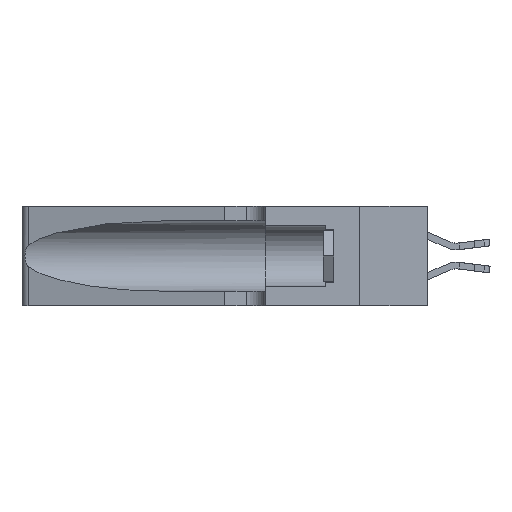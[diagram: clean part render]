
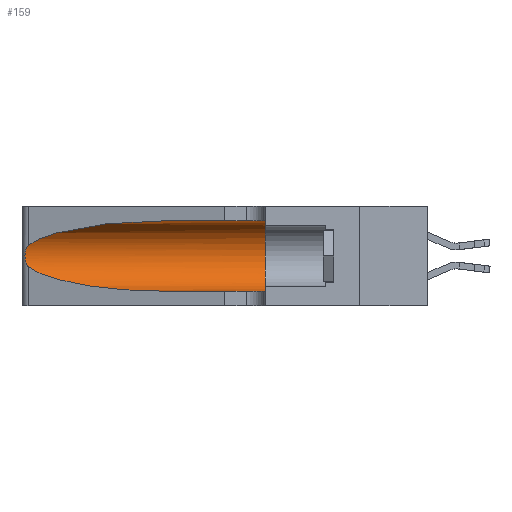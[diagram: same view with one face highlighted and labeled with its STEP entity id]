
A CAD part, left-side view. The second image highlights one B-rep face of the part: STEP entity #159.
In plain terms, the highlighted cylindrical face has radius 3.308 mm (diameter 6.617 mm), a partial arc.
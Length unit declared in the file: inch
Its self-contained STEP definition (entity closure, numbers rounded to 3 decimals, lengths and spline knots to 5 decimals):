
#159 = ADVANCED_FACE ( 'NONE', ( #13411 ), #8595, .F. ) ;
#199 = CARTESIAN_POINT ( 'NONE',  ( 0.1305, 0.35, 0.05475 ) ) ;
#634 = CARTESIAN_POINT ( 'NONE',  ( 0.26017, 1.23833, 0.17102 ) ) ;
#737 = CARTESIAN_POINT ( 'NONE',  ( 0.25487, 1.22718, 0.22369 ) ) ;
#1024 =( BOUNDED_CURVE ( )  B_SPLINE_CURVE ( 3, ( #13643, #17890, #12179, #4839 ),
 .UNSPECIFIED., .F., .T. ) 
 B_SPLINE_CURVE_WITH_KNOTS ( ( 4, 4 ),
 ( 3.44316, 4.71239 ),
 .UNSPECIFIED. ) 
 CURVE ( )  GEOMETRIC_REPRESENTATION_ITEM ( )  RATIONAL_B_SPLINE_CURVE ( ( 1., 0.87, 0.87, 1. ) ) 
 REPRESENTATION_ITEM ( '' )  );
#2103 = CARTESIAN_POINT ( 'NONE',  ( 0.25487, 1.22718, 0.22369 ) ) ;
#2173 = CARTESIAN_POINT ( 'NONE',  ( 0.25555, 1.22994, 0.2215 ) ) ;
#2237 = CARTESIAN_POINT ( 'NONE',  ( 0.25789, 1.23486, 0.15765 ) ) ;
#2696 = EDGE_CURVE ( 'NONE', #3798, #12055, #2937, .T. ) ;
#2868 = DIRECTION ( 'NONE',  ( 0., 1., 0. ) ) ;
#2937 =( BOUNDED_CURVE ( )  B_SPLINE_CURVE ( 3, ( #15737, #5533, #4028, #7050 ),
 .UNSPECIFIED., .F., .F. ) 
 B_SPLINE_CURVE_WITH_KNOTS ( ( 4, 4 ),
 ( 1.5708, 2.84003 ),
 .UNSPECIFIED. ) 
 CURVE ( )  GEOMETRIC_REPRESENTATION_ITEM ( )  RATIONAL_B_SPLINE_CURVE ( ( 1., 0.87, 0.87, 1. ) ) 
 REPRESENTATION_ITEM ( '' )  );
#3325 = VECTOR ( 'NONE', #5271, 39.37008 ) ;
#3624 = EDGE_CURVE ( 'NONE', #12443, #8370, #1024, .T. ) ;
#3798 = VERTEX_POINT ( 'NONE', #6885 ) ;
#3834 = CARTESIAN_POINT ( 'NONE',  ( 0.25555, 1.22993, 0.14849 ) ) ;
#4028 = CARTESIAN_POINT ( 'NONE',  ( 0.2373, 1.15595, 0.28018 ) ) ;
#4427 = EDGE_CURVE ( 'NONE', #12055, #12443, #14696, .T. ) ;
#4839 = CARTESIAN_POINT ( 'NONE',  ( 0.1305, 0.72297, 0.05475 ) ) ;
#5271 = DIRECTION ( 'NONE',  ( 0., -1., 0. ) ) ;
#5533 = CARTESIAN_POINT ( 'NONE',  ( 0.18966, 0.96281, 0.31525 ) ) ;
#5988 = AXIS2_PLACEMENT_3D ( 'NONE', #7553, #13206, #16961 ) ;
#6084 = CARTESIAN_POINT ( 'NONE',  ( 0.1305, 1.61858, 0.05475 ) ) ;
#6460 = EDGE_CURVE ( 'NONE', #8370, #10790, #11278, .T. ) ;
#6661 = ORIENTED_EDGE ( 'NONE', *, *, #2696, .T. ) ;
#6793 = CARTESIAN_POINT ( 'NONE',  ( 0.25787, 1.23484, 0.2124 ) ) ;
#6885 = CARTESIAN_POINT ( 'NONE',  ( 0.1305, 0.72297, 0.31525 ) ) ;
#6924 = ORIENTED_EDGE ( 'NONE', *, *, #4427, .T. ) ;
#6976 = ORIENTED_EDGE ( 'NONE', *, *, #3624, .T. ) ;
#7050 = CARTESIAN_POINT ( 'NONE',  ( 0.25487, 1.22718, 0.22369 ) ) ;
#7472 = AXIS2_PLACEMENT_3D ( 'NONE', #11776, #2868, #13247 ) ;
#7485 = ORIENTED_EDGE ( 'NONE', *, *, #8399, .F. ) ;
#7553 = CARTESIAN_POINT ( 'NONE',  ( 0.1305, 1.61858, 0.185 ) ) ;
#7874 = ORIENTED_EDGE ( 'NONE', *, *, #6460, .T. ) ;
#7990 = ORIENTED_EDGE ( 'NONE', *, *, #12810, .F. ) ;
#8241 = CARTESIAN_POINT ( 'NONE',  ( 0.26018, 1.23835, 0.19895 ) ) ;
#8370 = VERTEX_POINT ( 'NONE', #18313 ) ;
#8399 = EDGE_CURVE ( 'NONE', #3798, #17094, #15078, .T. ) ;
#8595 = CYLINDRICAL_SURFACE ( 'NONE', #5988, 0.13025 ) ;
#9730 = CARTESIAN_POINT ( 'NONE',  ( 0.26075, 1.23896, 0.178 ) ) ;
#10790 = VERTEX_POINT ( 'NONE', #199 ) ;
#10812 = VECTOR ( 'NONE', #17688, 39.37008 ) ;
#11194 = CARTESIAN_POINT ( 'NONE',  ( 0.25856, 1.23593, 0.16098 ) ) ;
#11278 = LINE ( 'NONE', #6084, #10812 ) ;
#11776 = CARTESIAN_POINT ( 'NONE',  ( 0.1305, 0.35, 0.185 ) ) ;
#12055 = VERTEX_POINT ( 'NONE', #737 ) ;
#12179 = CARTESIAN_POINT ( 'NONE',  ( 0.18966, 0.96281, 0.05475 ) ) ;
#12443 = VERTEX_POINT ( 'NONE', #15069 ) ;
#12680 = CARTESIAN_POINT ( 'NONE',  ( 0.25639, 1.23186, 0.15144 ) ) ;
#12705 = CIRCLE ( 'NONE', #7472, 0.13025 ) ;
#12810 = EDGE_CURVE ( 'NONE', #17094, #10790, #12705, .T. ) ;
#12853 = EDGE_LOOP ( 'NONE', ( #6661, #6924, #6976, #7874, #7990, #7485 ) ) ;
#13206 = DIRECTION ( 'NONE',  ( 0., -1., 0. ) ) ;
#13247 = DIRECTION ( 'NONE',  ( 0., 0., 1. ) ) ;
#13411 = FACE_OUTER_BOUND ( 'NONE', #12853, .T. ) ;
#13643 = CARTESIAN_POINT ( 'NONE',  ( 0.25487, 1.22718, 0.14631 ) ) ;
#14133 = CARTESIAN_POINT ( 'NONE',  ( 0.1305, 1.61858, 0.31525 ) ) ;
#14135 = CARTESIAN_POINT ( 'NONE',  ( 0.25487, 1.22718, 0.14631 ) ) ;
#14696 = B_SPLINE_CURVE_WITH_KNOTS ( 'NONE', 3,
 ( #2103, #2173, #15487, #6793, #16938, #8241, #18379, #9730, #634, #11194, #2237, #12680, #3834, #14135 ),
 .UNSPECIFIED., .F., .F.,
 ( 4, 2, 2, 2, 2, 2, 4 ),
 ( 0., 0.00027, 0.00053, 0.00107, 0.0016, 0.00187, 0.00214 ),
 .UNSPECIFIED. ) ;
#15069 = CARTESIAN_POINT ( 'NONE',  ( 0.25487, 1.22718, 0.14631 ) ) ;
#15078 = LINE ( 'NONE', #14133, #3325 ) ;
#15487 = CARTESIAN_POINT ( 'NONE',  ( 0.25639, 1.23184, 0.21858 ) ) ;
#15737 = CARTESIAN_POINT ( 'NONE',  ( 0.1305, 0.72297, 0.31525 ) ) ;
#16938 = CARTESIAN_POINT ( 'NONE',  ( 0.25854, 1.2359, 0.20912 ) ) ;
#16961 = DIRECTION ( 'NONE',  ( 0., 0., -1. ) ) ;
#17094 = VERTEX_POINT ( 'NONE', #17643 ) ;
#17643 = CARTESIAN_POINT ( 'NONE',  ( 0.1305, 0.35, 0.31525 ) ) ;
#17688 = DIRECTION ( 'NONE',  ( 0., -1., 0. ) ) ;
#17890 = CARTESIAN_POINT ( 'NONE',  ( 0.2373, 1.15595, 0.08982 ) ) ;
#18313 = CARTESIAN_POINT ( 'NONE',  ( 0.1305, 0.72297, 0.05475 ) ) ;
#18379 = CARTESIAN_POINT ( 'NONE',  ( 0.26075, 1.23896, 0.19203 ) ) ;
